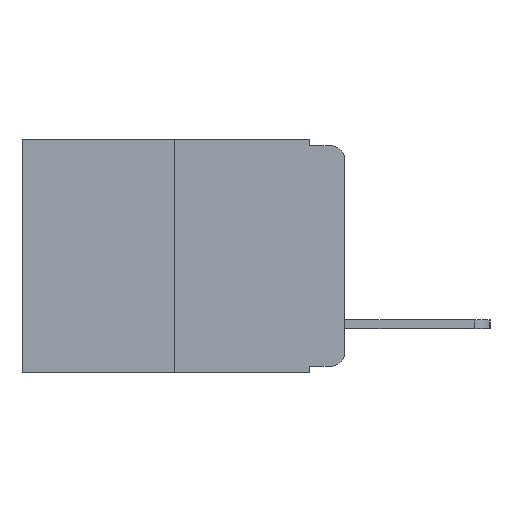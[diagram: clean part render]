
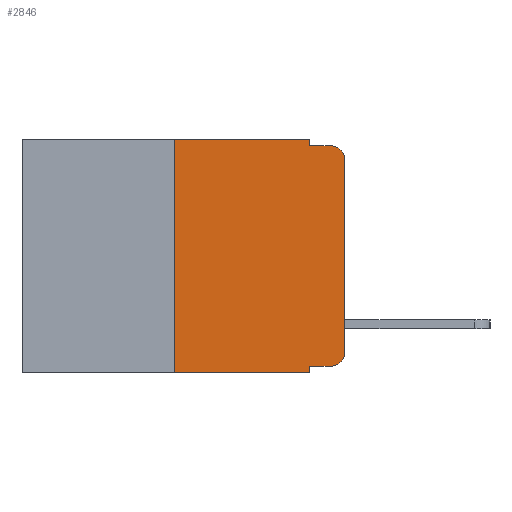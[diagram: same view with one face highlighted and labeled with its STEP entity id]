
A CAD part, left-side view. The second image highlights one B-rep face of the part: STEP entity #2846.
In plain terms, the highlighted planar face has unit normal (-1, 0, 0).
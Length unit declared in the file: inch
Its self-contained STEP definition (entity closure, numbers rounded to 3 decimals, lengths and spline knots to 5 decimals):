
#70 = VECTOR ( 'NONE', #11668, 39.37008 ) ;
#413 = FACE_OUTER_BOUND ( 'NONE', #13870, .T. ) ;
#434 = EDGE_CURVE ( 'NONE', #10806, #11096, #12110, .T. ) ;
#729 = VECTOR ( 'NONE', #21448, 39.37008 ) ;
#931 = EDGE_CURVE ( 'NONE', #13673, #16820, #19546, .T. ) ;
#1497 = CARTESIAN_POINT ( 'NONE',  ( 0., 0., -0.313 ) ) ;
#1654 = DIRECTION ( 'NONE',  ( 0., 0., -1. ) ) ;
#1717 = ORIENTED_EDGE ( 'NONE', *, *, #14665, .T. ) ;
#1758 = ORIENTED_EDGE ( 'NONE', *, *, #434, .T. ) ;
#1771 = ORIENTED_EDGE ( 'NONE', *, *, #20496, .F. ) ;
#1862 = ORIENTED_EDGE ( 'NONE', *, *, #17244, .F. ) ;
#2268 = VECTOR ( 'NONE', #1654, 39.37008 ) ;
#2361 = AXIS2_PLACEMENT_3D ( 'NONE', #10676, #10632, #9378 ) ;
#2368 = ORIENTED_EDGE ( 'NONE', *, *, #2863, .F. ) ;
#2500 = ORIENTED_EDGE ( 'NONE', *, *, #6064, .F. ) ;
#2530 = CARTESIAN_POINT ( 'NONE',  ( 0., 0.051, -0.343 ) ) ;
#2846 = ADVANCED_FACE ( 'NONE', ( #413 ), #17856, .F. ) ;
#2863 = EDGE_CURVE ( 'NONE', #7183, #18526, #9108, .T. ) ;
#2985 = EDGE_CURVE ( 'NONE', #3147, #16820, #4696, .T. ) ;
#3147 = VERTEX_POINT ( 'NONE', #15825 ) ;
#3163 = ORIENTED_EDGE ( 'NONE', *, *, #2985, .T. ) ;
#3221 = CARTESIAN_POINT ( 'NONE',  ( 0., 0.25, 0. ) ) ;
#3229 = VECTOR ( 'NONE', #17355, 39.37008 ) ;
#4175 = ORIENTED_EDGE ( 'NONE', *, *, #931, .F. ) ;
#4696 = LINE ( 'NONE', #11685, #70 ) ;
#4841 = CARTESIAN_POINT ( 'NONE',  ( 0., 0.051, -0.333 ) ) ;
#5128 = ORIENTED_EDGE ( 'NONE', *, *, #21945, .T. ) ;
#5643 = CARTESIAN_POINT ( 'NONE',  ( 0., 0., 0. ) ) ;
#6064 = EDGE_CURVE ( 'NONE', #3147, #7183, #15203, .T. ) ;
#6241 = ORIENTED_EDGE ( 'NONE', *, *, #19837, .T. ) ;
#6763 = CARTESIAN_POINT ( 'NONE',  ( 0., 0.02, -0.313 ) ) ;
#7183 = VERTEX_POINT ( 'NONE', #15512 ) ;
#7298 = CARTESIAN_POINT ( 'NONE',  ( 0., 0.02, -0.01 ) ) ;
#7963 = LINE ( 'NONE', #4841, #16259 ) ;
#8546 = DIRECTION ( 'NONE',  ( 0., 0., -1. ) ) ;
#9108 = LINE ( 'NONE', #17080, #17851 ) ;
#9378 = DIRECTION ( 'NONE',  ( 0., 0., -1. ) ) ;
#10300 = VECTOR ( 'NONE', #16890, 39.37008 ) ;
#10632 = DIRECTION ( 'NONE',  ( -1., 0., 0. ) ) ;
#10676 = CARTESIAN_POINT ( 'NONE',  ( 0., 0.02, -0.03 ) ) ;
#10806 = VERTEX_POINT ( 'NONE', #19940 ) ;
#11096 = VERTEX_POINT ( 'NONE', #7298 ) ;
#11668 = DIRECTION ( 'NONE',  ( 0., -1., 0. ) ) ;
#11685 = CARTESIAN_POINT ( 'NONE',  ( 0., 0.473, -0.343 ) ) ;
#11773 = CARTESIAN_POINT ( 'NONE',  ( 0., 0.02, -0.333 ) ) ;
#12110 = CIRCLE ( 'NONE', #2361, 0.02 ) ;
#12154 = LINE ( 'NONE', #12230, #2268 ) ;
#12230 = CARTESIAN_POINT ( 'NONE',  ( 0., 0.051, 0. ) ) ;
#12260 = AXIS2_PLACEMENT_3D ( 'NONE', #17673, #17650, #17632 ) ;
#13213 = DIRECTION ( 'NONE',  ( 0., 0., -1. ) ) ;
#13257 = CARTESIAN_POINT ( 'NONE',  ( 0., 0.051, 0. ) ) ;
#13428 = VERTEX_POINT ( 'NONE', #16958 ) ;
#13495 = CARTESIAN_POINT ( 'NONE',  ( 0., 0.051, 0. ) ) ;
#13673 = VERTEX_POINT ( 'NONE', #20684 ) ;
#13870 = EDGE_LOOP ( 'NONE', ( #1717, #1758, #1771, #1862, #2368, #2500, #3163, #4175, #5128, #6241 ) ) ;
#14277 = LINE ( 'NONE', #19870, #729 ) ;
#14665 = EDGE_CURVE ( 'NONE', #16278, #10806, #16870, .T. ) ;
#15203 = LINE ( 'NONE', #3221, #10300 ) ;
#15233 = VECTOR ( 'NONE', #13213, 39.37008 ) ;
#15512 = CARTESIAN_POINT ( 'NONE',  ( 0., 0.25, 0. ) ) ;
#15825 = CARTESIAN_POINT ( 'NONE',  ( 0., 0.25, -0.343 ) ) ;
#15829 = CIRCLE ( 'NONE', #21247, 0.02 ) ;
#16259 = VECTOR ( 'NONE', #16574, 39.37008 ) ;
#16278 = VERTEX_POINT ( 'NONE', #1497 ) ;
#16574 = DIRECTION ( 'NONE',  ( 0., -1., 0. ) ) ;
#16820 = VERTEX_POINT ( 'NONE', #2530 ) ;
#16870 = LINE ( 'NONE', #5643, #3229 ) ;
#16890 = DIRECTION ( 'NONE',  ( 0., 0., 1. ) ) ;
#16958 = CARTESIAN_POINT ( 'NONE',  ( 0., 0.051, -0.01 ) ) ;
#17080 = CARTESIAN_POINT ( 'NONE',  ( 0., 0.473, 0. ) ) ;
#17244 = EDGE_CURVE ( 'NONE', #18526, #13428, #12154, .T. ) ;
#17355 = DIRECTION ( 'NONE',  ( 0., 0., 1. ) ) ;
#17632 = DIRECTION ( 'NONE',  ( 0., 0., -1. ) ) ;
#17650 = DIRECTION ( 'NONE',  ( 1., 0., 0. ) ) ;
#17673 = CARTESIAN_POINT ( 'NONE',  ( 0., 0.473, 0. ) ) ;
#17851 = VECTOR ( 'NONE', #19318, 39.37008 ) ;
#17856 = PLANE ( 'NONE',  #12260 ) ;
#18393 = DIRECTION ( 'NONE',  ( -1., 0., 0. ) ) ;
#18526 = VERTEX_POINT ( 'NONE', #13495 ) ;
#19318 = DIRECTION ( 'NONE',  ( 0., -1., 0. ) ) ;
#19546 = LINE ( 'NONE', #13257, #15233 ) ;
#19818 = VERTEX_POINT ( 'NONE', #11773 ) ;
#19837 = EDGE_CURVE ( 'NONE', #19818, #16278, #15829, .T. ) ;
#19870 = CARTESIAN_POINT ( 'NONE',  ( 0., 0.051, -0.01 ) ) ;
#19940 = CARTESIAN_POINT ( 'NONE',  ( 0., 0., -0.03 ) ) ;
#20496 = EDGE_CURVE ( 'NONE', #13428, #11096, #14277, .T. ) ;
#20684 = CARTESIAN_POINT ( 'NONE',  ( 0., 0.051, -0.333 ) ) ;
#21247 = AXIS2_PLACEMENT_3D ( 'NONE', #6763, #18393, #8546 ) ;
#21448 = DIRECTION ( 'NONE',  ( 0., -1., 0. ) ) ;
#21945 = EDGE_CURVE ( 'NONE', #13673, #19818, #7963, .T. ) ;
